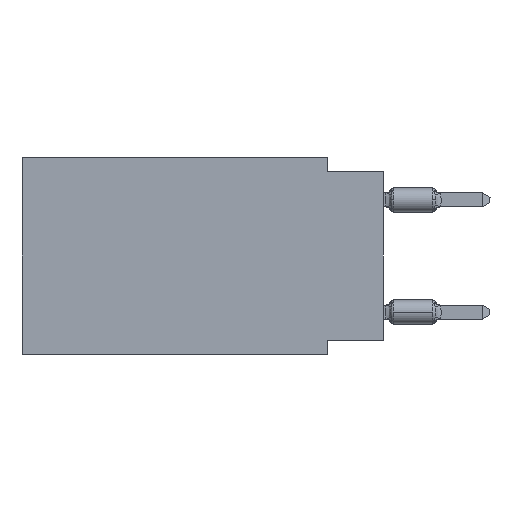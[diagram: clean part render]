
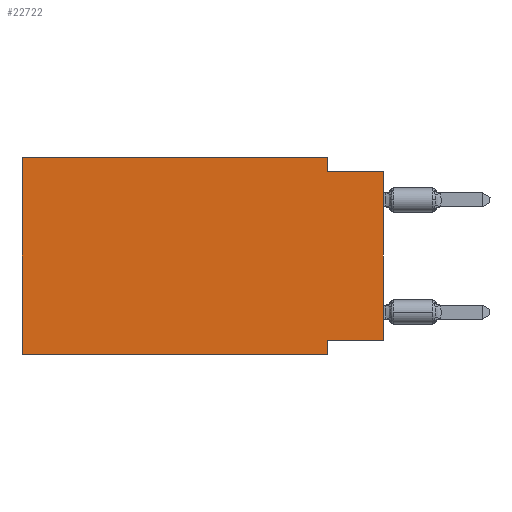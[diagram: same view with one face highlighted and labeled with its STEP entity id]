
A CAD part, left-side view. The second image highlights one B-rep face of the part: STEP entity #22722.
In plain terms, the highlighted planar face has unit normal (-1, 0, 0).
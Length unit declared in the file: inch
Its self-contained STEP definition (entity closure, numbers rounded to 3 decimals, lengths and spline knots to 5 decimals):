
#1571 = VECTOR ( 'NONE', #27681, 39.37008 ) ;
#2379 = VERTEX_POINT ( 'NONE', #49520 ) ;
#2857 = VERTEX_POINT ( 'NONE', #15187 ) ;
#5545 = EDGE_CURVE ( 'NONE', #43175, #52123, #14642, .T. ) ;
#6832 = LINE ( 'NONE', #26756, #10199 ) ;
#6945 = LINE ( 'NONE', #37344, #1571 ) ;
#7094 = LINE ( 'NONE', #20099, #10339 ) ;
#7605 = ORIENTED_EDGE ( 'NONE', *, *, #5545, .F. ) ;
#8991 = DIRECTION ( 'NONE',  ( 0., 0., -1. ) ) ;
#9023 = VECTOR ( 'NONE', #39245, 39.37008 ) ;
#9220 = LINE ( 'NONE', #43249, #42104 ) ;
#10199 = VECTOR ( 'NONE', #27832, 39.37008 ) ;
#10339 = VECTOR ( 'NONE', #36670, 39.37008 ) ;
#10785 = DIRECTION ( 'NONE',  ( 0., 1., 0. ) ) ;
#12536 = ORIENTED_EDGE ( 'NONE', *, *, #38295, .F. ) ;
#12999 = ORIENTED_EDGE ( 'NONE', *, *, #13286, .T. ) ;
#13286 = EDGE_CURVE ( 'NONE', #26306, #52123, #9220, .T. ) ;
#14642 = LINE ( 'NONE', #17978, #9023 ) ;
#15111 = EDGE_CURVE ( 'NONE', #16557, #43175, #54395, .T. ) ;
#15187 = CARTESIAN_POINT ( 'NONE',  ( 0., 0.1, 0. ) ) ;
#15410 = LINE ( 'NONE', #52732, #21622 ) ;
#16557 = VERTEX_POINT ( 'NONE', #25689 ) ;
#16964 = ORIENTED_EDGE ( 'NONE', *, *, #42391, .F. ) ;
#17978 = CARTESIAN_POINT ( 'NONE',  ( 0., 0.1, -0.35 ) ) ;
#18734 = EDGE_CURVE ( 'NONE', #52394, #2857, #44663, .T. ) ;
#18823 = CARTESIAN_POINT ( 'NONE',  ( 0., 0., -0.325 ) ) ;
#19406 = CARTESIAN_POINT ( 'NONE',  ( 0., 0.1, -0.025 ) ) ;
#20099 = CARTESIAN_POINT ( 'NONE',  ( 0., 0., -0.025 ) ) ;
#20962 = ORIENTED_EDGE ( 'NONE', *, *, #34180, .F. ) ;
#21622 = VECTOR ( 'NONE', #36402, 39.37008 ) ;
#22277 = FACE_OUTER_BOUND ( 'NONE', #40473, .T. ) ;
#22588 = ORIENTED_EDGE ( 'NONE', *, *, #15111, .F. ) ;
#22722 = ADVANCED_FACE ( 'NONE', ( #22277 ), #25583, .F. ) ;
#25356 = CARTESIAN_POINT ( 'NONE',  ( 0., 0.645, 0. ) ) ;
#25583 = PLANE ( 'NONE',  #35013 ) ;
#25689 = CARTESIAN_POINT ( 'NONE',  ( 0., 0., -0.325 ) ) ;
#26052 = ORIENTED_EDGE ( 'NONE', *, *, #18734, .F. ) ;
#26306 = VERTEX_POINT ( 'NONE', #29742 ) ;
#26756 = CARTESIAN_POINT ( 'NONE',  ( 0., 0., 0. ) ) ;
#27365 = CARTESIAN_POINT ( 'NONE',  ( 0., 0.1, -0.325 ) ) ;
#27681 = DIRECTION ( 'NONE',  ( 0., 0., 1. ) ) ;
#27832 = DIRECTION ( 'NONE',  ( 0., 0., 1. ) ) ;
#29742 = CARTESIAN_POINT ( 'NONE',  ( 0., 0.645, -0.35 ) ) ;
#34180 = EDGE_CURVE ( 'NONE', #2857, #36947, #15410, .T. ) ;
#34587 = ORIENTED_EDGE ( 'NONE', *, *, #46101, .T. ) ;
#35013 = AXIS2_PLACEMENT_3D ( 'NONE', #46870, #51583, #8991 ) ;
#36354 = CARTESIAN_POINT ( 'NONE',  ( 0., 0.645, 0. ) ) ;
#36402 = DIRECTION ( 'NONE',  ( 0., 0., -1. ) ) ;
#36670 = DIRECTION ( 'NONE',  ( 0., -1., 0. ) ) ;
#36947 = VERTEX_POINT ( 'NONE', #19406 ) ;
#37344 = CARTESIAN_POINT ( 'NONE',  ( 0., 0.645, 0. ) ) ;
#38295 = EDGE_CURVE ( 'NONE', #26306, #52394, #6945, .T. ) ;
#38530 = DIRECTION ( 'NONE',  ( 0., -1., 0. ) ) ;
#39245 = DIRECTION ( 'NONE',  ( 0., 0., -1. ) ) ;
#40473 = EDGE_LOOP ( 'NONE', ( #34587, #16964, #20962, #26052, #12536, #12999, #7605, #22588 ) ) ;
#42104 = VECTOR ( 'NONE', #38530, 39.37008 ) ;
#42391 = EDGE_CURVE ( 'NONE', #36947, #2379, #7094, .T. ) ;
#43175 = VERTEX_POINT ( 'NONE', #27365 ) ;
#43249 = CARTESIAN_POINT ( 'NONE',  ( 0., 0.645, -0.35 ) ) ;
#44663 = LINE ( 'NONE', #36354, #46562 ) ;
#46101 = EDGE_CURVE ( 'NONE', #16557, #2379, #6832, .T. ) ;
#46562 = VECTOR ( 'NONE', #53778, 39.37008 ) ;
#46870 = CARTESIAN_POINT ( 'NONE',  ( 0., 0.645, 0. ) ) ;
#48219 = VECTOR ( 'NONE', #10785, 39.37008 ) ;
#49520 = CARTESIAN_POINT ( 'NONE',  ( 0., 0., -0.025 ) ) ;
#51583 = DIRECTION ( 'NONE',  ( 1., 0., 0. ) ) ;
#52123 = VERTEX_POINT ( 'NONE', #52506 ) ;
#52394 = VERTEX_POINT ( 'NONE', #25356 ) ;
#52506 = CARTESIAN_POINT ( 'NONE',  ( 0., 0.1, -0.35 ) ) ;
#52732 = CARTESIAN_POINT ( 'NONE',  ( 0., 0.1, 0. ) ) ;
#53778 = DIRECTION ( 'NONE',  ( 0., -1., 0. ) ) ;
#54395 = LINE ( 'NONE', #18823, #48219 ) ;
